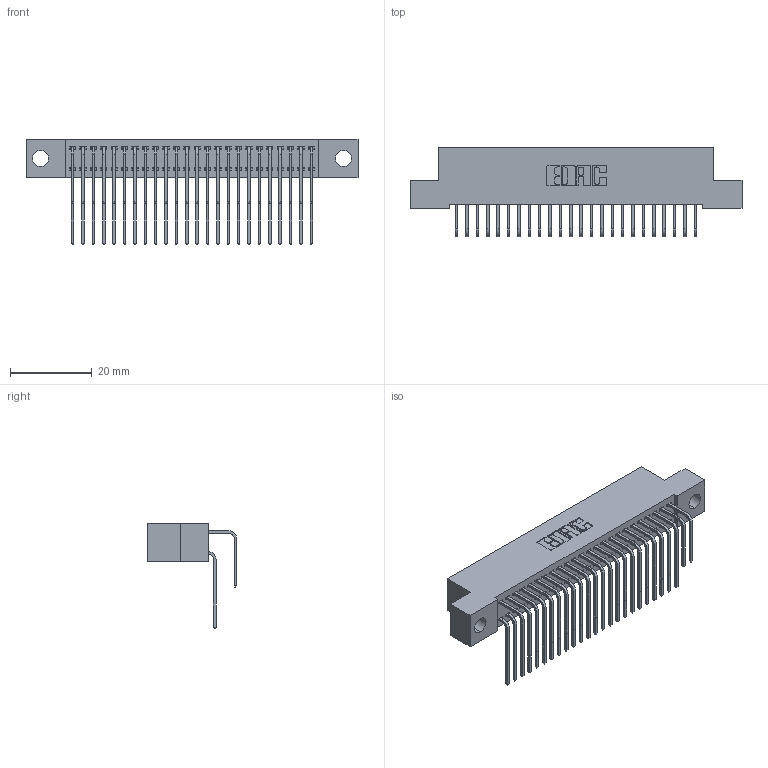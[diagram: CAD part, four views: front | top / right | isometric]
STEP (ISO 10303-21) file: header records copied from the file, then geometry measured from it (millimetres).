
FILE_DESCRIPTION (( 'STEP AP203' ), '1' );
FILE_NAME ('342-048-558-204.STEP', '2019-10-02T22:27:57', ( '' ), ( '' ), 'SwSTEP 2.0', 'SolidWorks 2016', '' );
FILE_SCHEMA (( 'CONFIG_CONTROL_DESIGN' ));
Length unit declared in the file: inch
Products named in the file (4): 342 Part_.156 TH; 345-292-001_558 559 Tail - 1; 345-292-001_558 Tail - 2; 342-048-558-204
Assembly tree (49 placements, depth 2):
  342-048-558-204
    342 Part_.156 TH
    345-292-001_558 559 Tail - 1  x24
    345-292-001_558 Tail - 2  x24
Bounding box: 81.28 x 21.91 x 25.78 mm (x, y, z)
Volume: 7407.7 mm3; surface area: 12691.1 mm2
Topology: 49 solids, 49 shells, 2702 faces, 8027 edges, 5286 vertices
Faces by surface type: plane 1890, cylinder 812
Entity records: 19423 total; most frequent: CARTESIAN_POINT 3289, ORIENTED_EDGE 3174, DIRECTION 2823, EDGE_CURVE 1587, VECTOR 1419, LINE 1419, VERTEX_POINT 1054, AXIS2_PLACEMENT_3D 702
